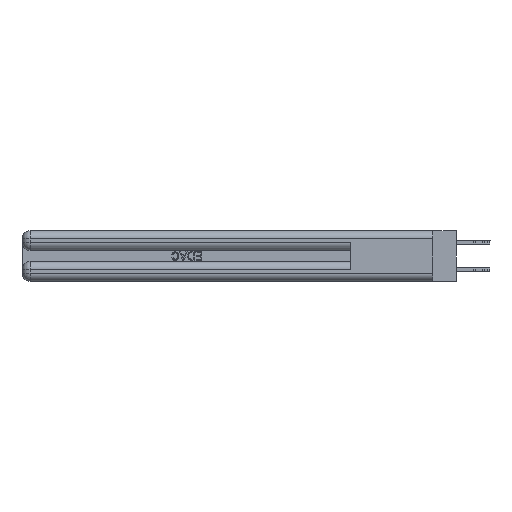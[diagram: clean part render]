
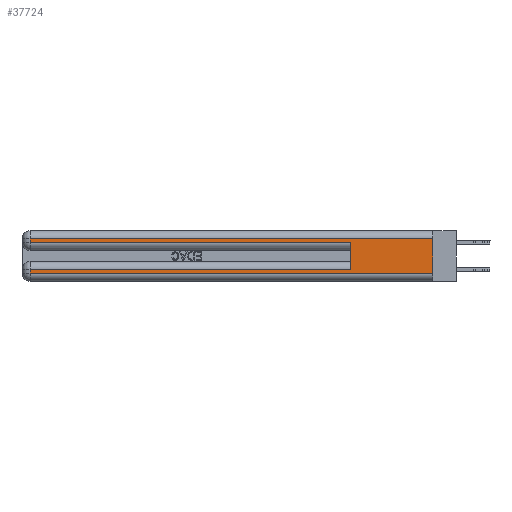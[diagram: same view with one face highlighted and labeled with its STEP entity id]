
A CAD part, left-side view. The second image highlights one B-rep face of the part: STEP entity #37724.
In plain terms, the highlighted planar face has unit normal (-1, 0, 0).
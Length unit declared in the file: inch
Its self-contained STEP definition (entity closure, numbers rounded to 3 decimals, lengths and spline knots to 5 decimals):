
#74 = EDGE_CURVE ( 'NONE', #41490, #37878, #41766, .T. ) ;
#532 = EDGE_CURVE ( 'NONE', #38948, #8113, #13349, .T. ) ;
#994 = EDGE_LOOP ( 'NONE', ( #5016, #38963, #10073, #39275, #15469, #13663, #9729, #12646 ) ) ;
#2546 = EDGE_CURVE ( 'NONE', #6084, #36779, #27281, .T. ) ;
#3338 = CARTESIAN_POINT ( 'NONE',  ( 0., 0., 0.085 ) ) ;
#3684 = LINE ( 'NONE', #21348, #29102 ) ;
#3715 = CARTESIAN_POINT ( 'NONE',  ( 0., 0., 0.31 ) ) ;
#4036 = CARTESIAN_POINT ( 'NONE',  ( 0., 2.94, 0.06 ) ) ;
#4091 = DIRECTION ( 'NONE',  ( 0., -1., 0. ) ) ;
#4561 = CARTESIAN_POINT ( 'NONE',  ( 0., 2.94, 0.285 ) ) ;
#5016 = ORIENTED_EDGE ( 'NONE', *, *, #28791, .F. ) ;
#6084 = VERTEX_POINT ( 'NONE', #4036 ) ;
#7596 = DIRECTION ( 'NONE',  ( 0., 0., -1. ) ) ;
#8096 = VERTEX_POINT ( 'NONE', #4561 ) ;
#8113 = VERTEX_POINT ( 'NONE', #17505 ) ;
#8738 = VECTOR ( 'NONE', #24281, 39.37008 ) ;
#9667 = LINE ( 'NONE', #22312, #30856 ) ;
#9729 = ORIENTED_EDGE ( 'NONE', *, *, #29038, .T. ) ;
#10073 = ORIENTED_EDGE ( 'NONE', *, *, #10188, .T. ) ;
#10188 = EDGE_CURVE ( 'NONE', #8113, #8096, #26343, .T. ) ;
#10920 = DIRECTION ( 'NONE',  ( 0., -1., 0. ) ) ;
#12646 = ORIENTED_EDGE ( 'NONE', *, *, #2546, .T. ) ;
#12869 = DIRECTION ( 'NONE',  ( 0., 1., 0. ) ) ;
#13349 = LINE ( 'NONE', #32000, #35641 ) ;
#13663 = ORIENTED_EDGE ( 'NONE', *, *, #74, .T. ) ;
#14094 = CARTESIAN_POINT ( 'NONE',  ( 0., 0., 0.285 ) ) ;
#15469 = ORIENTED_EDGE ( 'NONE', *, *, #25890, .F. ) ;
#17505 = CARTESIAN_POINT ( 'NONE',  ( 0., 2.94, 0.31 ) ) ;
#19049 = CARTESIAN_POINT ( 'NONE',  ( 0., 0., 0.37 ) ) ;
#19713 = FACE_OUTER_BOUND ( 'NONE', #994, .T. ) ;
#19859 = CARTESIAN_POINT ( 'NONE',  ( 0., 2.94, 0.085 ) ) ;
#20565 = CARTESIAN_POINT ( 'NONE',  ( 0., 2.94, 0.37 ) ) ;
#21348 = CARTESIAN_POINT ( 'NONE',  ( 0., 0.6, 0.145 ) ) ;
#22312 = CARTESIAN_POINT ( 'NONE',  ( 0., 0., 0.37 ) ) ;
#22738 = DIRECTION ( 'NONE',  ( 0., 0., -1. ) ) ;
#23207 = VECTOR ( 'NONE', #23281, 39.37008 ) ;
#23281 = DIRECTION ( 'NONE',  ( 0., 1., 0. ) ) ;
#23669 = CARTESIAN_POINT ( 'NONE',  ( 0., 0., 0.06 ) ) ;
#24110 = VECTOR ( 'NONE', #10920, 39.37008 ) ;
#24281 = DIRECTION ( 'NONE',  ( 0., 0., -1. ) ) ;
#25890 = EDGE_CURVE ( 'NONE', #41490, #30220, #3684, .T. ) ;
#26343 = LINE ( 'NONE', #20565, #8738 ) ;
#27007 = LINE ( 'NONE', #14094, #37869 ) ;
#27013 = CARTESIAN_POINT ( 'NONE',  ( 0., 0.6, 0.285 ) ) ;
#27281 = LINE ( 'NONE', #23669, #24110 ) ;
#28312 = DIRECTION ( 'NONE',  ( 1., 0., 0. ) ) ;
#28791 = EDGE_CURVE ( 'NONE', #38948, #36779, #9667, .T. ) ;
#29038 = EDGE_CURVE ( 'NONE', #37878, #6084, #35990, .T. ) ;
#29102 = VECTOR ( 'NONE', #31196, 39.37008 ) ;
#30220 = VERTEX_POINT ( 'NONE', #27013 ) ;
#30314 = VECTOR ( 'NONE', #7596, 39.37008 ) ;
#30389 = CARTESIAN_POINT ( 'NONE',  ( 0., 0., 0.06 ) ) ;
#30782 = EDGE_CURVE ( 'NONE', #8096, #30220, #27007, .T. ) ;
#30856 = VECTOR ( 'NONE', #22738, 39.37008 ) ;
#31196 = DIRECTION ( 'NONE',  ( 0., 0., 1. ) ) ;
#31403 = CARTESIAN_POINT ( 'NONE',  ( 0., 0.6, 0.085 ) ) ;
#32000 = CARTESIAN_POINT ( 'NONE',  ( 0., 0., 0.31 ) ) ;
#32665 = AXIS2_PLACEMENT_3D ( 'NONE', #19049, #28312, #38676 ) ;
#33490 = CARTESIAN_POINT ( 'NONE',  ( 0., 2.94, 0.37 ) ) ;
#35641 = VECTOR ( 'NONE', #12869, 39.37008 ) ;
#35990 = LINE ( 'NONE', #33490, #30314 ) ;
#36779 = VERTEX_POINT ( 'NONE', #30389 ) ;
#37724 = ADVANCED_FACE ( 'NONE', ( #19713 ), #38806, .F. ) ;
#37869 = VECTOR ( 'NONE', #4091, 39.37008 ) ;
#37878 = VERTEX_POINT ( 'NONE', #19859 ) ;
#38676 = DIRECTION ( 'NONE',  ( 0., 0., -1. ) ) ;
#38806 = PLANE ( 'NONE',  #32665 ) ;
#38948 = VERTEX_POINT ( 'NONE', #3715 ) ;
#38963 = ORIENTED_EDGE ( 'NONE', *, *, #532, .T. ) ;
#39275 = ORIENTED_EDGE ( 'NONE', *, *, #30782, .T. ) ;
#41490 = VERTEX_POINT ( 'NONE', #31403 ) ;
#41766 = LINE ( 'NONE', #3338, #23207 ) ;
